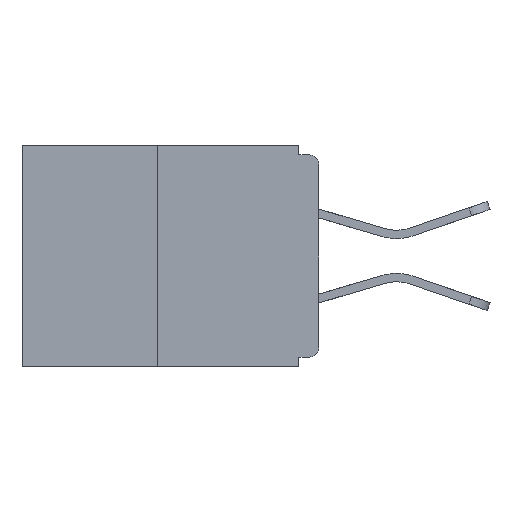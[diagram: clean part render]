
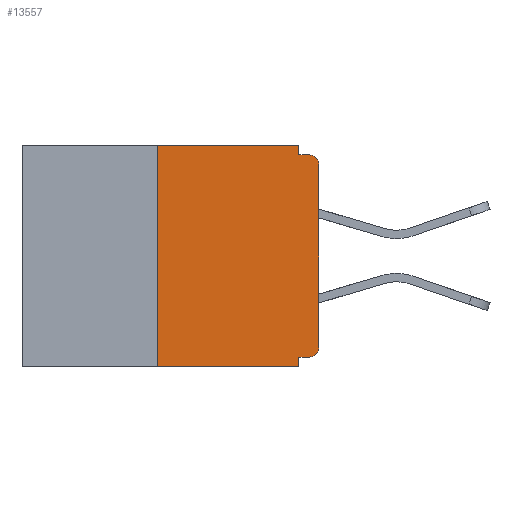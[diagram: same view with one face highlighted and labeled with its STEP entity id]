
A CAD part, left-side view. The second image highlights one B-rep face of the part: STEP entity #13557.
In plain terms, the highlighted planar face has unit normal (-1, 0, 0).
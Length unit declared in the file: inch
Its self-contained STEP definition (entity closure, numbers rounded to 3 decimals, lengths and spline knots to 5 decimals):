
#93 = VERTEX_POINT ( 'NONE', #5642 ) ;
#154 = VERTEX_POINT ( 'NONE', #4383 ) ;
#184 = DIRECTION ( 'NONE',  ( 0., 0., 1. ) ) ;
#720 = VECTOR ( 'NONE', #8195, 39.37008 ) ;
#992 = CARTESIAN_POINT ( 'NONE',  ( 0., 0.46, 0. ) ) ;
#1342 = ORIENTED_EDGE ( 'NONE', *, *, #13212, .F. ) ;
#1377 = ORIENTED_EDGE ( 'NONE', *, *, #10970, .F. ) ;
#1594 = DIRECTION ( 'NONE',  ( -1., 0., 0. ) ) ;
#1615 = AXIS2_PLACEMENT_3D ( 'NONE', #2770, #1594, #8768 ) ;
#2173 = CARTESIAN_POINT ( 'NONE',  ( 0., 0.015, -0.328 ) ) ;
#2342 = EDGE_CURVE ( 'NONE', #8191, #15226, #4702, .T. ) ;
#2741 = VECTOR ( 'NONE', #14223, 39.37008 ) ;
#2770 = CARTESIAN_POINT ( 'NONE',  ( 0., 0.015, -0.313 ) ) ;
#2970 = VERTEX_POINT ( 'NONE', #12730 ) ;
#3190 = CARTESIAN_POINT ( 'NONE',  ( 0., 0.46, 0. ) ) ;
#3210 = CARTESIAN_POINT ( 'NONE',  ( 0., 0.031, -0.343 ) ) ;
#3275 = DIRECTION ( 'NONE',  ( 0., 1., 0. ) ) ;
#3403 = FACE_OUTER_BOUND ( 'NONE', #13459, .T. ) ;
#3868 = LINE ( 'NONE', #3210, #9793 ) ;
#4304 = LINE ( 'NONE', #5045, #12693 ) ;
#4370 = DIRECTION ( 'NONE',  ( 0., 0., -1. ) ) ;
#4383 = CARTESIAN_POINT ( 'NONE',  ( 0., 0.25, 0. ) ) ;
#4400 = DIRECTION ( 'NONE',  ( 0., 0., -1. ) ) ;
#4483 = ORIENTED_EDGE ( 'NONE', *, *, #9528, .T. ) ;
#4487 = VECTOR ( 'NONE', #5730, 39.37008 ) ;
#4565 = EDGE_CURVE ( 'NONE', #2970, #93, #3868, .T. ) ;
#4581 = CARTESIAN_POINT ( 'NONE',  ( 0., 0.015, -0.03 ) ) ;
#4702 = CIRCLE ( 'NONE', #9487, 0.015 ) ;
#4868 = LINE ( 'NONE', #992, #720 ) ;
#5045 = CARTESIAN_POINT ( 'NONE',  ( 0., 0., 0. ) ) ;
#5115 = CARTESIAN_POINT ( 'NONE',  ( 0., 0.015, -0.015 ) ) ;
#5642 = CARTESIAN_POINT ( 'NONE',  ( 0., 0.031, -0.343 ) ) ;
#5667 = LINE ( 'NONE', #6989, #11797 ) ;
#5730 = DIRECTION ( 'NONE',  ( 0., 0., 1. ) ) ;
#5798 = CARTESIAN_POINT ( 'NONE',  ( 0., 0., -0.03 ) ) ;
#6036 = VECTOR ( 'NONE', #6117, 39.37008 ) ;
#6115 = LINE ( 'NONE', #10606, #2741 ) ;
#6117 = DIRECTION ( 'NONE',  ( 0., -1., 0. ) ) ;
#6989 = CARTESIAN_POINT ( 'NONE',  ( 0., 0., -0.328 ) ) ;
#7031 = ORIENTED_EDGE ( 'NONE', *, *, #7087, .T. ) ;
#7087 = EDGE_CURVE ( 'NONE', #8322, #8191, #4304, .T. ) ;
#7793 = ORIENTED_EDGE ( 'NONE', *, *, #15319, .F. ) ;
#7873 = ORIENTED_EDGE ( 'NONE', *, *, #9257, .T. ) ;
#7965 = EDGE_CURVE ( 'NONE', #9323, #9236, #12857, .T. ) ;
#8108 = CARTESIAN_POINT ( 'NONE',  ( 0., 0.031, -0.015 ) ) ;
#8191 = VERTEX_POINT ( 'NONE', #5798 ) ;
#8195 = DIRECTION ( 'NONE',  ( 0., -1., 0. ) ) ;
#8322 = VERTEX_POINT ( 'NONE', #15378 ) ;
#8352 = ORIENTED_EDGE ( 'NONE', *, *, #7965, .F. ) ;
#8691 = CARTESIAN_POINT ( 'NONE',  ( 0., 0., -0.015 ) ) ;
#8768 = DIRECTION ( 'NONE',  ( 0., 0., -1. ) ) ;
#8957 = CARTESIAN_POINT ( 'NONE',  ( 0., 0.25, -0.343 ) ) ;
#9236 = VERTEX_POINT ( 'NONE', #8108 ) ;
#9257 = EDGE_CURVE ( 'NONE', #11696, #93, #6115, .T. ) ;
#9322 = LINE ( 'NONE', #8691, #6036 ) ;
#9323 = VERTEX_POINT ( 'NONE', #13958 ) ;
#9487 = AXIS2_PLACEMENT_3D ( 'NONE', #4581, #11659, #4370 ) ;
#9528 = EDGE_CURVE ( 'NONE', #10063, #8322, #15294, .T. ) ;
#9615 = VECTOR ( 'NONE', #9959, 39.37008 ) ;
#9793 = VECTOR ( 'NONE', #14174, 39.37008 ) ;
#9959 = DIRECTION ( 'NONE',  ( 0., 0., -1. ) ) ;
#10063 = VERTEX_POINT ( 'NONE', #2173 ) ;
#10114 = AXIS2_PLACEMENT_3D ( 'NONE', #3190, #11691, #4400 ) ;
#10606 = CARTESIAN_POINT ( 'NONE',  ( 0., 0.46, -0.343 ) ) ;
#10623 = CARTESIAN_POINT ( 'NONE',  ( 0., 0.25, 0. ) ) ;
#10970 = EDGE_CURVE ( 'NONE', #10063, #2970, #5667, .T. ) ;
#11170 = LINE ( 'NONE', #10623, #4487 ) ;
#11659 = DIRECTION ( 'NONE',  ( -1., 0., 0. ) ) ;
#11691 = DIRECTION ( 'NONE',  ( 1., 0., 0. ) ) ;
#11696 = VERTEX_POINT ( 'NONE', #8957 ) ;
#11797 = VECTOR ( 'NONE', #3275, 39.37008 ) ;
#12361 = CARTESIAN_POINT ( 'NONE',  ( 0., 0.031, 0. ) ) ;
#12693 = VECTOR ( 'NONE', #184, 39.37008 ) ;
#12730 = CARTESIAN_POINT ( 'NONE',  ( 0., 0.031, -0.328 ) ) ;
#12857 = LINE ( 'NONE', #12361, #9615 ) ;
#12985 = ORIENTED_EDGE ( 'NONE', *, *, #4565, .F. ) ;
#13212 = EDGE_CURVE ( 'NONE', #9236, #15226, #9322, .T. ) ;
#13459 = EDGE_LOOP ( 'NONE', ( #7793, #15303, #7873, #12985, #1377, #4483, #7031, #13530, #1342, #8352 ) ) ;
#13530 = ORIENTED_EDGE ( 'NONE', *, *, #2342, .T. ) ;
#13557 = ADVANCED_FACE ( 'NONE', ( #3403 ), #15455, .F. ) ;
#13958 = CARTESIAN_POINT ( 'NONE',  ( 0., 0.031, 0. ) ) ;
#14174 = DIRECTION ( 'NONE',  ( 0., 0., -1. ) ) ;
#14223 = DIRECTION ( 'NONE',  ( 0., -1., 0. ) ) ;
#15226 = VERTEX_POINT ( 'NONE', #5115 ) ;
#15294 = CIRCLE ( 'NONE', #1615, 0.015 ) ;
#15303 = ORIENTED_EDGE ( 'NONE', *, *, #15341, .F. ) ;
#15319 = EDGE_CURVE ( 'NONE', #154, #9323, #4868, .T. ) ;
#15341 = EDGE_CURVE ( 'NONE', #11696, #154, #11170, .T. ) ;
#15378 = CARTESIAN_POINT ( 'NONE',  ( 0., 0., -0.313 ) ) ;
#15455 = PLANE ( 'NONE',  #10114 ) ;
